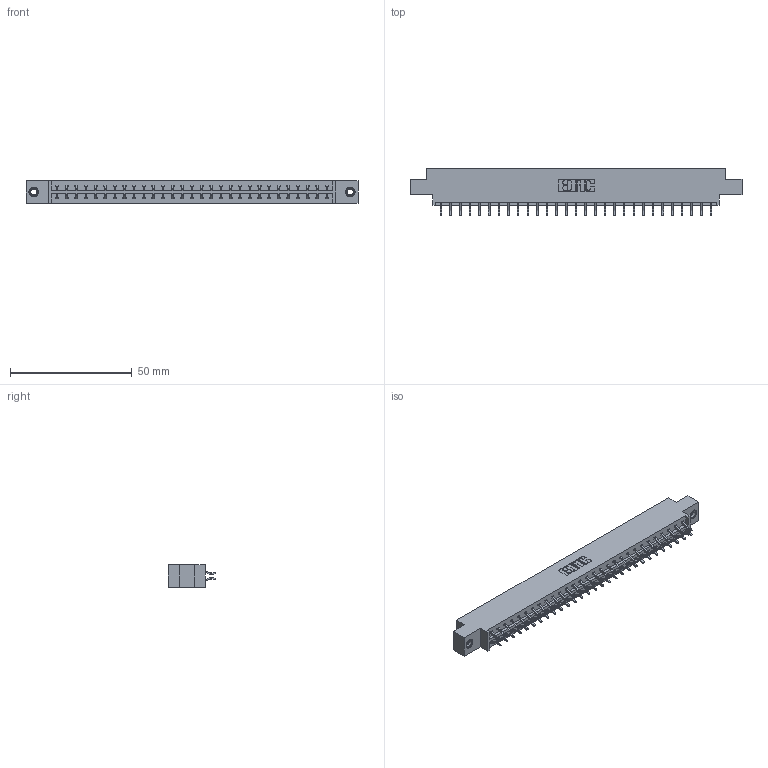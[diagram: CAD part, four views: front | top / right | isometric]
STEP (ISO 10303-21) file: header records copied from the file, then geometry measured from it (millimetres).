
FILE_DESCRIPTION (( 'STEP AP203' ), '1' );
FILE_NAME ('333-058-556-807.STEP', '2018-08-04T06:25:26', ( '' ), ( '' ), 'SwSTEP 2.0', 'SolidWorks 2016', '' );
FILE_SCHEMA (( 'CONFIG_CONTROL_DESIGN' ));
Length unit declared in the file: inch
Products named in the file (4): 345-292-001_556 Tail; 345-250-001_345-250-005-103; 333-058-556-807; 333 Part_Offset - .156 Dia - TI
Assembly tree (61 placements, depth 2):
  333-058-556-807
    333 Part_Offset - .156 Dia - TI
    345-292-001_556 Tail  x58
    345-250-001_345-250-005-103  x2
Bounding box: 136.45 x 19.57 x 9.4 mm (x, y, z)
Volume: 13565.5 mm3; surface area: 16095.8 mm2
Topology: 61 solids, 61 shells, 3542 faces, 10493 edges, 6910 vertices
Faces by surface type: plane 2426, cylinder 1100, cone 12, torus 4
Entity records: 21876 total; most frequent: CARTESIAN_POINT 3641, ORIENTED_EDGE 3558, DIRECTION 3153, EDGE_CURVE 1779, LINE 1623, VECTOR 1623, VERTEX_POINT 1180, AXIS2_PLACEMENT_3D 765
